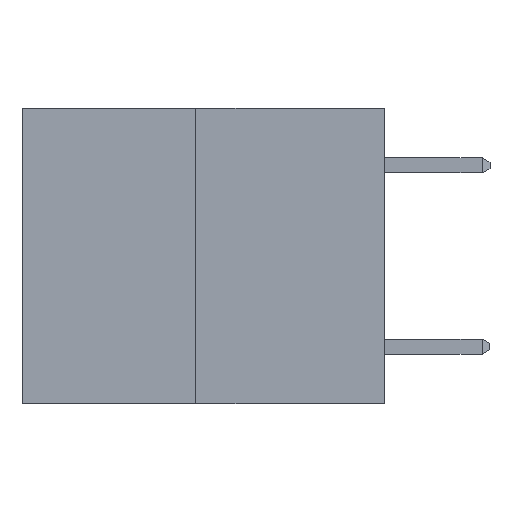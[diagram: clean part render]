
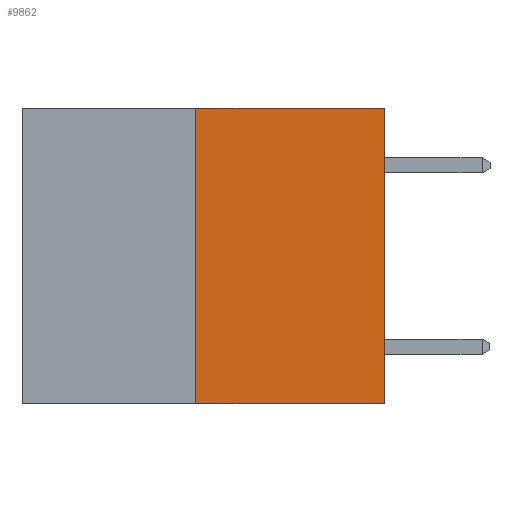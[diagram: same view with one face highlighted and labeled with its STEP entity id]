
A CAD part, left-side view. The second image highlights one B-rep face of the part: STEP entity #9862.
In plain terms, the highlighted planar face has unit normal (-1, 0, 0).
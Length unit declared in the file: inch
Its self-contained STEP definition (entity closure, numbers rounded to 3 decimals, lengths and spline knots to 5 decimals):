
#104 = LINE ( 'NONE', #9951, #17051 ) ;
#743 = CARTESIAN_POINT ( 'NONE',  ( 0., 0.312, 0. ) ) ;
#901 = EDGE_CURVE ( 'NONE', #8339, #11341, #104, .T. ) ;
#2848 = LINE ( 'NONE', #10527, #9571 ) ;
#4166 = VECTOR ( 'NONE', #14639, 39.37008 ) ;
#4511 = DIRECTION ( 'NONE',  ( 0., 0., -1. ) ) ;
#4767 = ORIENTED_EDGE ( 'NONE', *, *, #12304, .F. ) ;
#5857 = LINE ( 'NONE', #15216, #14816 ) ;
#7099 = CARTESIAN_POINT ( 'NONE',  ( 0., 0.6, 0. ) ) ;
#8210 = CARTESIAN_POINT ( 'NONE',  ( 0., 0.6, 0. ) ) ;
#8339 = VERTEX_POINT ( 'NONE', #12342 ) ;
#8928 = VERTEX_POINT ( 'NONE', #743 ) ;
#9448 = PLANE ( 'NONE',  #9902 ) ;
#9571 = VECTOR ( 'NONE', #15098, 39.37008 ) ;
#9862 = ADVANCED_FACE ( 'NONE', ( #18062 ), #9448, .F. ) ;
#9902 = AXIS2_PLACEMENT_3D ( 'NONE', #7099, #16830, #4511 ) ;
#9951 = CARTESIAN_POINT ( 'NONE',  ( 0., 0., 0. ) ) ;
#10527 = CARTESIAN_POINT ( 'NONE',  ( 0., 0.312, -0.49 ) ) ;
#10657 = LINE ( 'NONE', #8210, #4166 ) ;
#11332 = VERTEX_POINT ( 'NONE', #16458 ) ;
#11341 = VERTEX_POINT ( 'NONE', #16525 ) ;
#11744 = ORIENTED_EDGE ( 'NONE', *, *, #15239, .F. ) ;
#12304 = EDGE_CURVE ( 'NONE', #8928, #11341, #10657, .T. ) ;
#12342 = CARTESIAN_POINT ( 'NONE',  ( 0., 0., -0.49 ) ) ;
#13492 = ORIENTED_EDGE ( 'NONE', *, *, #901, .T. ) ;
#14639 = DIRECTION ( 'NONE',  ( 0., -1., 0. ) ) ;
#14816 = VECTOR ( 'NONE', #15148, 39.37008 ) ;
#15098 = DIRECTION ( 'NONE',  ( 0., 0., 1. ) ) ;
#15148 = DIRECTION ( 'NONE',  ( 0., -1., 0. ) ) ;
#15216 = CARTESIAN_POINT ( 'NONE',  ( 0., 0.6, -0.49 ) ) ;
#15239 = EDGE_CURVE ( 'NONE', #11332, #8928, #2848, .T. ) ;
#15496 = DIRECTION ( 'NONE',  ( 0., 0., 1. ) ) ;
#16458 = CARTESIAN_POINT ( 'NONE',  ( 0., 0.312, -0.49 ) ) ;
#16525 = CARTESIAN_POINT ( 'NONE',  ( 0., 0., 0. ) ) ;
#16581 = ORIENTED_EDGE ( 'NONE', *, *, #17881, .T. ) ;
#16830 = DIRECTION ( 'NONE',  ( 1., 0., 0. ) ) ;
#17051 = VECTOR ( 'NONE', #15496, 39.37008 ) ;
#17125 = EDGE_LOOP ( 'NONE', ( #11744, #16581, #13492, #4767 ) ) ;
#17881 = EDGE_CURVE ( 'NONE', #11332, #8339, #5857, .T. ) ;
#18062 = FACE_OUTER_BOUND ( 'NONE', #17125, .T. ) ;
